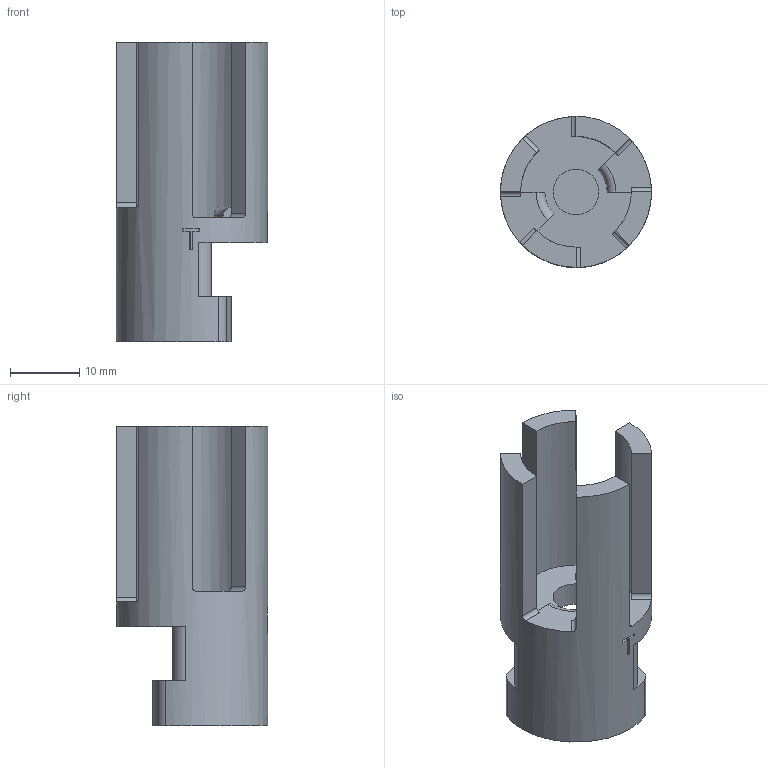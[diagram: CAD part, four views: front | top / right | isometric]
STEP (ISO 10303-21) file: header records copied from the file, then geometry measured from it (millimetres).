
FILE_DESCRIPTION(/* description */ (''),/* implementation_level */ '2;1');
FILE_NAME(/* name */ 'Throating End Pilot Inch (0.250in).stp',/* time_stamp */ '2021-02-15T01:55:54-06:00',/* author */ ('johne'),/* organization */ (''),/* preprocessor_version */ 'ST-DEVELOPER v18',/* originating_system */ 'Autodesk Inventor 2020',/* authorisation */ '');
FILE_SCHEMA (('AUTOMOTIVE_DESIGN { 1 0 10303 214 3 1 1 }'));
Length unit declared in the file: millimetre
Products named in the file (1): Throating Tool 250 rod
Bounding box: 21.84 x 21.84 x 43.36 mm (x, y, z)
Volume: 5744.2 mm3; surface area: 4052.7 mm2
Topology: 1 solids, 1 shells, 55 faces, 156 edges, 104 vertices
Faces by surface type: plane 31, cylinder 22, torus 2
Full cylindrical faces by diameter (mm): 6.604 x1, 21.844 x1
Entity records: 1963 total; most frequent: CARTESIAN_POINT 460, ORIENTED_EDGE 312, DIRECTION 308, EDGE_CURVE 156, AXIS2_PLACEMENT_3D 112, VERTEX_POINT 104, LINE 84, VECTOR 84
